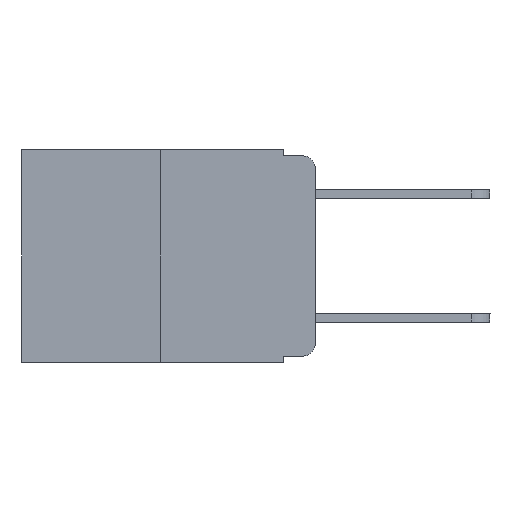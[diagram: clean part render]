
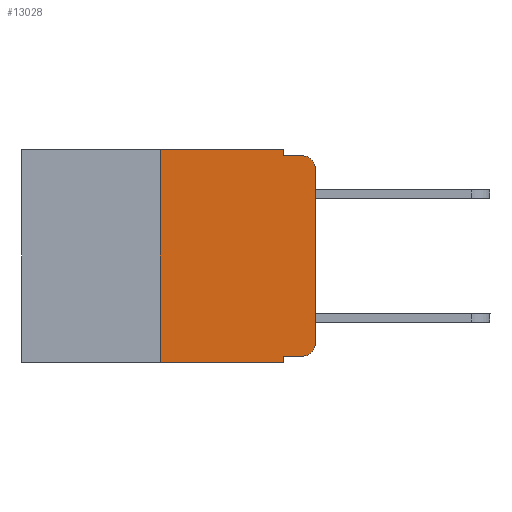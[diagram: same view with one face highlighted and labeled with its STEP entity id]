
A CAD part, left-side view. The second image highlights one B-rep face of the part: STEP entity #13028.
In plain terms, the highlighted planar face has unit normal (-1, 0, 0).
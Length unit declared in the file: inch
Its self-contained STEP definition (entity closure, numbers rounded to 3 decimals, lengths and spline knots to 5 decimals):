
#385 = CARTESIAN_POINT ( 'NONE',  ( 0., 0.051, -0.333 ) ) ;
#495 = CARTESIAN_POINT ( 'NONE',  ( 0., 0.02, -0.333 ) ) ;
#524 = LINE ( 'NONE', #385, #12248 ) ;
#565 = ORIENTED_EDGE ( 'NONE', *, *, #19155, .F. ) ;
#671 = CIRCLE ( 'NONE', #5939, 0.02 ) ;
#780 = EDGE_CURVE ( 'NONE', #15300, #7504, #3023, .T. ) ;
#844 = CARTESIAN_POINT ( 'NONE',  ( 0., 0.02, -0.01 ) ) ;
#904 = DIRECTION ( 'NONE',  ( 1., 0., 0. ) ) ;
#955 = ORIENTED_EDGE ( 'NONE', *, *, #3641, .T. ) ;
#1743 = LINE ( 'NONE', #9681, #3650 ) ;
#1762 = EDGE_CURVE ( 'NONE', #11025, #2680, #671, .T. ) ;
#1836 = EDGE_LOOP ( 'NONE', ( #4095, #7181, #565, #13689, #17582, #6072, #955, #4850, #7797, #6404 ) ) ;
#2361 = CARTESIAN_POINT ( 'NONE',  ( 0., 0.051, -0.333 ) ) ;
#2429 = VERTEX_POINT ( 'NONE', #19067 ) ;
#2554 = CARTESIAN_POINT ( 'NONE',  ( 0., 0.25, 0. ) ) ;
#2680 = VERTEX_POINT ( 'NONE', #9114 ) ;
#2984 = LINE ( 'NONE', #2554, #12287 ) ;
#3023 = CIRCLE ( 'NONE', #4105, 0.02 ) ;
#3207 = VECTOR ( 'NONE', #15125, 39.37008 ) ;
#3571 = EDGE_CURVE ( 'NONE', #2429, #19087, #12761, .T. ) ;
#3641 = EDGE_CURVE ( 'NONE', #13560, #16215, #19178, .T. ) ;
#3650 = VECTOR ( 'NONE', #18838, 39.37008 ) ;
#4072 = DIRECTION ( 'NONE',  ( 0., 0., 1. ) ) ;
#4095 = ORIENTED_EDGE ( 'NONE', *, *, #4467, .T. ) ;
#4105 = AXIS2_PLACEMENT_3D ( 'NONE', #9313, #4749, #12421 ) ;
#4131 = DIRECTION ( 'NONE',  ( 0., 0., -1. ) ) ;
#4467 = EDGE_CURVE ( 'NONE', #2680, #15300, #1743, .T. ) ;
#4749 = DIRECTION ( 'NONE',  ( -1., 0., 0. ) ) ;
#4771 = EDGE_CURVE ( 'NONE', #7884, #11025, #524, .T. ) ;
#4850 = ORIENTED_EDGE ( 'NONE', *, *, #14284, .F. ) ;
#5143 = VECTOR ( 'NONE', #9191, 39.37008 ) ;
#5939 = AXIS2_PLACEMENT_3D ( 'NONE', #18229, #12261, #6065 ) ;
#6065 = DIRECTION ( 'NONE',  ( 0., 0., -1. ) ) ;
#6072 = ORIENTED_EDGE ( 'NONE', *, *, #17810, .F. ) ;
#6404 = ORIENTED_EDGE ( 'NONE', *, *, #1762, .T. ) ;
#6792 = CARTESIAN_POINT ( 'NONE',  ( 0., 0.051, -0.343 ) ) ;
#7011 = EDGE_CURVE ( 'NONE', #19087, #12210, #15708, .T. ) ;
#7181 = ORIENTED_EDGE ( 'NONE', *, *, #780, .T. ) ;
#7308 = CARTESIAN_POINT ( 'NONE',  ( 0., 0., -0.03 ) ) ;
#7504 = VERTEX_POINT ( 'NONE', #844 ) ;
#7732 = DIRECTION ( 'NONE',  ( 0., -1., 0. ) ) ;
#7797 = ORIENTED_EDGE ( 'NONE', *, *, #4771, .T. ) ;
#7884 = VERTEX_POINT ( 'NONE', #2361 ) ;
#8128 = VECTOR ( 'NONE', #4131, 39.37008 ) ;
#8432 = VECTOR ( 'NONE', #10918, 39.37008 ) ;
#9114 = CARTESIAN_POINT ( 'NONE',  ( 0., 0., -0.313 ) ) ;
#9191 = DIRECTION ( 'NONE',  ( 0., -1., 0. ) ) ;
#9313 = CARTESIAN_POINT ( 'NONE',  ( 0., 0.02, -0.03 ) ) ;
#9314 = CARTESIAN_POINT ( 'NONE',  ( 0., 0.473, -0.343 ) ) ;
#9681 = CARTESIAN_POINT ( 'NONE',  ( 0., 0., 0. ) ) ;
#10243 = CARTESIAN_POINT ( 'NONE',  ( 0., 0.25, -0.343 ) ) ;
#10597 = CARTESIAN_POINT ( 'NONE',  ( 0., 0.051, 0. ) ) ;
#10730 = CARTESIAN_POINT ( 'NONE',  ( 0., 0.051, 0. ) ) ;
#10781 = CARTESIAN_POINT ( 'NONE',  ( 0., 0.051, -0.01 ) ) ;
#10808 = LINE ( 'NONE', #10730, #8432 ) ;
#10889 = DIRECTION ( 'NONE',  ( 0., -1., 0. ) ) ;
#10918 = DIRECTION ( 'NONE',  ( 0., 0., -1. ) ) ;
#11025 = VERTEX_POINT ( 'NONE', #495 ) ;
#11597 = DIRECTION ( 'NONE',  ( 0., 0., -1. ) ) ;
#12210 = VERTEX_POINT ( 'NONE', #12829 ) ;
#12248 = VECTOR ( 'NONE', #10889, 39.37008 ) ;
#12261 = DIRECTION ( 'NONE',  ( -1., 0., 0. ) ) ;
#12287 = VECTOR ( 'NONE', #4072, 39.37008 ) ;
#12421 = DIRECTION ( 'NONE',  ( 0., 0., -1. ) ) ;
#12761 = LINE ( 'NONE', #18262, #3207 ) ;
#12829 = CARTESIAN_POINT ( 'NONE',  ( 0., 0.051, -0.01 ) ) ;
#12974 = AXIS2_PLACEMENT_3D ( 'NONE', #17539, #904, #11597 ) ;
#13000 = FACE_OUTER_BOUND ( 'NONE', #1836, .T. ) ;
#13028 = ADVANCED_FACE ( 'NONE', ( #13000 ), #19146, .F. ) ;
#13560 = VERTEX_POINT ( 'NONE', #10243 ) ;
#13689 = ORIENTED_EDGE ( 'NONE', *, *, #7011, .F. ) ;
#14284 = EDGE_CURVE ( 'NONE', #7884, #16215, #10808, .T. ) ;
#15125 = DIRECTION ( 'NONE',  ( 0., -1., 0. ) ) ;
#15300 = VERTEX_POINT ( 'NONE', #7308 ) ;
#15708 = LINE ( 'NONE', #19571, #8128 ) ;
#16215 = VERTEX_POINT ( 'NONE', #6792 ) ;
#16497 = LINE ( 'NONE', #10781, #18635 ) ;
#17539 = CARTESIAN_POINT ( 'NONE',  ( 0., 0.473, 0. ) ) ;
#17582 = ORIENTED_EDGE ( 'NONE', *, *, #3571, .F. ) ;
#17810 = EDGE_CURVE ( 'NONE', #13560, #2429, #2984, .T. ) ;
#18229 = CARTESIAN_POINT ( 'NONE',  ( 0., 0.02, -0.313 ) ) ;
#18262 = CARTESIAN_POINT ( 'NONE',  ( 0., 0.473, 0. ) ) ;
#18635 = VECTOR ( 'NONE', #7732, 39.37008 ) ;
#18838 = DIRECTION ( 'NONE',  ( 0., 0., 1. ) ) ;
#19067 = CARTESIAN_POINT ( 'NONE',  ( 0., 0.25, 0. ) ) ;
#19087 = VERTEX_POINT ( 'NONE', #10597 ) ;
#19146 = PLANE ( 'NONE',  #12974 ) ;
#19155 = EDGE_CURVE ( 'NONE', #12210, #7504, #16497, .T. ) ;
#19178 = LINE ( 'NONE', #9314, #5143 ) ;
#19571 = CARTESIAN_POINT ( 'NONE',  ( 0., 0.051, 0. ) ) ;
